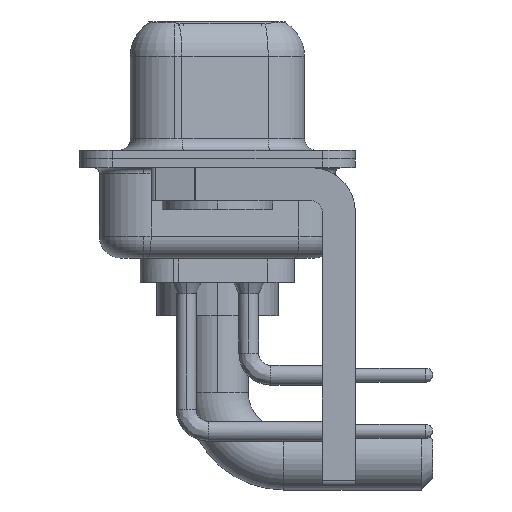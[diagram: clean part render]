
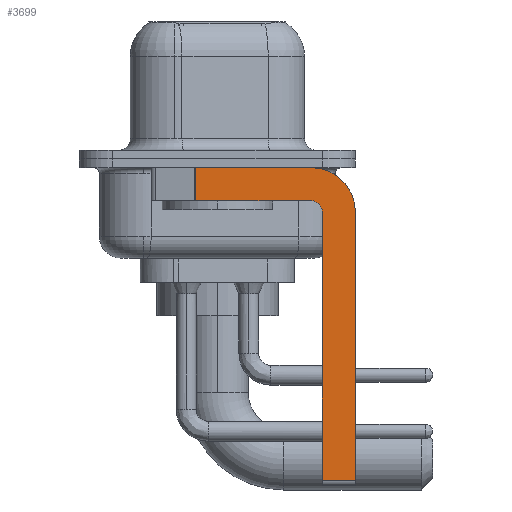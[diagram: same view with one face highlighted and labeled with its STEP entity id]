
A CAD part, left-side view. The second image highlights one B-rep face of the part: STEP entity #3699.
In plain terms, the highlighted planar face has unit normal (-1, 0, 0).
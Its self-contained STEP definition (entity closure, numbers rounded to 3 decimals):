
#90 = CARTESIAN_POINT ( 'NONE',  ( -2.9, -4.25, -1.9 ) ) ;
#191 = CARTESIAN_POINT ( 'NONE',  ( -2.9, -6.25, -14.55 ) ) ;
#614 = VERTEX_POINT ( 'NONE', #4441 ) ;
#788 = VECTOR ( 'NONE', #1688, 1000. ) ;
#872 = ORIENTED_EDGE ( 'NONE', *, *, #13159, .F. ) ;
#1137 = CIRCLE ( 'NONE', #3033, 0.5 ) ;
#1588 = LINE ( 'NONE', #7589, #788 ) ;
#1688 = DIRECTION ( 'NONE',  ( 0., -1., 0. ) ) ;
#2909 = ORIENTED_EDGE ( 'NONE', *, *, #13926, .T. ) ;
#3033 = AXIS2_PLACEMENT_3D ( 'NONE', #8276, #18784, #18500 ) ;
#3699 = ADVANCED_FACE ( 'NONE', ( #5338 ), #11358, .F. ) ;
#3704 = LINE ( 'NONE', #17180, #15862 ) ;
#3710 = ORIENTED_EDGE ( 'NONE', *, *, #9432, .F. ) ;
#3969 = CARTESIAN_POINT ( 'NONE',  ( -2.9, 0.978, -1.9 ) ) ;
#4441 = CARTESIAN_POINT ( 'NONE',  ( -2.9, -4.75, -14.55 ) ) ;
#4621 = DIRECTION ( 'NONE',  ( 0., 0., 1. ) ) ;
#4712 = EDGE_CURVE ( 'NONE', #8459, #14004, #7225, .T. ) ;
#5014 = ORIENTED_EDGE ( 'NONE', *, *, #4712, .F. ) ;
#5274 = DIRECTION ( 'NONE',  ( 0., 0., -1. ) ) ;
#5338 = FACE_OUTER_BOUND ( 'NONE', #18023, .T. ) ;
#6114 = VECTOR ( 'NONE', #4621, 1000. ) ;
#6151 = DIRECTION ( 'NONE',  ( 0., -1., 0. ) ) ;
#6668 = ORIENTED_EDGE ( 'NONE', *, *, #17465, .F. ) ;
#6687 = VERTEX_POINT ( 'NONE', #13798 ) ;
#6974 = VECTOR ( 'NONE', #6151, 1000. ) ;
#7070 = EDGE_CURVE ( 'NONE', #614, #15176, #9069, .T. ) ;
#7104 = CARTESIAN_POINT ( 'NONE',  ( -2.9, -4.25, -2.4 ) ) ;
#7196 = DIRECTION ( 'NONE',  ( 1., 0., 0. ) ) ;
#7225 = LINE ( 'NONE', #13250, #6974 ) ;
#7589 = CARTESIAN_POINT ( 'NONE',  ( -2.9, -4.25, -14.55 ) ) ;
#7731 = CARTESIAN_POINT ( 'NONE',  ( -2.9, -6.25, -2.4 ) ) ;
#8137 = AXIS2_PLACEMENT_3D ( 'NONE', #9067, #16525, #13495 ) ;
#8276 = CARTESIAN_POINT ( 'NONE',  ( -2.9, -4.25, -2.4 ) ) ;
#8459 = VERTEX_POINT ( 'NONE', #12098 ) ;
#9067 = CARTESIAN_POINT ( 'NONE',  ( -2.9, -4.25, -2.4 ) ) ;
#9069 = LINE ( 'NONE', #19277, #6114 ) ;
#9432 = EDGE_CURVE ( 'NONE', #15176, #9752, #1137, .T. ) ;
#9752 = VERTEX_POINT ( 'NONE', #90 ) ;
#9984 = DIRECTION ( 'NONE',  ( 0., 0., -1. ) ) ;
#10027 = CIRCLE ( 'NONE', #8137, 2. ) ;
#10039 = ORIENTED_EDGE ( 'NONE', *, *, #7070, .F. ) ;
#10301 = ORIENTED_EDGE ( 'NONE', *, *, #12680, .T. ) ;
#11226 = CARTESIAN_POINT ( 'NONE',  ( -2.9, -4.25, -0.4 ) ) ;
#11358 = PLANE ( 'NONE',  #17303 ) ;
#11449 = DIRECTION ( 'NONE',  ( 0., 0., -1. ) ) ;
#12088 = LINE ( 'NONE', #17785, #17262 ) ;
#12098 = CARTESIAN_POINT ( 'NONE',  ( -2.9, 0.978, -0.4 ) ) ;
#12680 = EDGE_CURVE ( 'NONE', #8459, #6687, #15681, .T. ) ;
#13159 = EDGE_CURVE ( 'NONE', #14743, #16244, #3704, .T. ) ;
#13250 = CARTESIAN_POINT ( 'NONE',  ( -2.9, 3., -0.4 ) ) ;
#13495 = DIRECTION ( 'NONE',  ( 0., 0., -1. ) ) ;
#13798 = CARTESIAN_POINT ( 'NONE',  ( -2.9, 0.978, -1.9 ) ) ;
#13926 = EDGE_CURVE ( 'NONE', #614, #16244, #1588, .T. ) ;
#14004 = VERTEX_POINT ( 'NONE', #11226 ) ;
#14743 = VERTEX_POINT ( 'NONE', #7731 ) ;
#14895 = CARTESIAN_POINT ( 'NONE',  ( -2.9, -4.75, -2.4 ) ) ;
#15151 = ORIENTED_EDGE ( 'NONE', *, *, #17770, .F. ) ;
#15176 = VERTEX_POINT ( 'NONE', #14895 ) ;
#15268 = VECTOR ( 'NONE', #9984, 1000. ) ;
#15681 = LINE ( 'NONE', #3969, #15268 ) ;
#15862 = VECTOR ( 'NONE', #5274, 1000. ) ;
#16244 = VERTEX_POINT ( 'NONE', #191 ) ;
#16525 = DIRECTION ( 'NONE',  ( 1., 0., 0. ) ) ;
#17180 = CARTESIAN_POINT ( 'NONE',  ( -2.9, -6.25, -2.4 ) ) ;
#17262 = VECTOR ( 'NONE', #17883, 1000. ) ;
#17303 = AXIS2_PLACEMENT_3D ( 'NONE', #7104, #7196, #11449 ) ;
#17465 = EDGE_CURVE ( 'NONE', #14004, #14743, #10027, .T. ) ;
#17770 = EDGE_CURVE ( 'NONE', #9752, #6687, #12088, .T. ) ;
#17785 = CARTESIAN_POINT ( 'NONE',  ( -2.9, -4.25, -1.9 ) ) ;
#17883 = DIRECTION ( 'NONE',  ( 0., 1., 0. ) ) ;
#18023 = EDGE_LOOP ( 'NONE', ( #5014, #10301, #15151, #3710, #10039, #2909, #872, #6668 ) ) ;
#18500 = DIRECTION ( 'NONE',  ( 0., 0., 1. ) ) ;
#18784 = DIRECTION ( 'NONE',  ( -1., 0., 0. ) ) ;
#19277 = CARTESIAN_POINT ( 'NONE',  ( -2.9, -4.75, -14.8 ) ) ;
